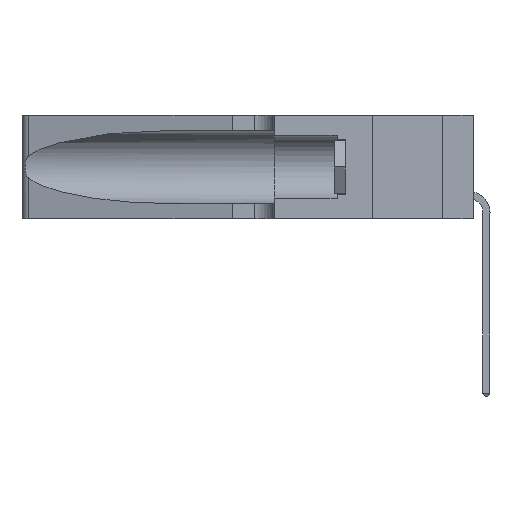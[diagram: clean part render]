
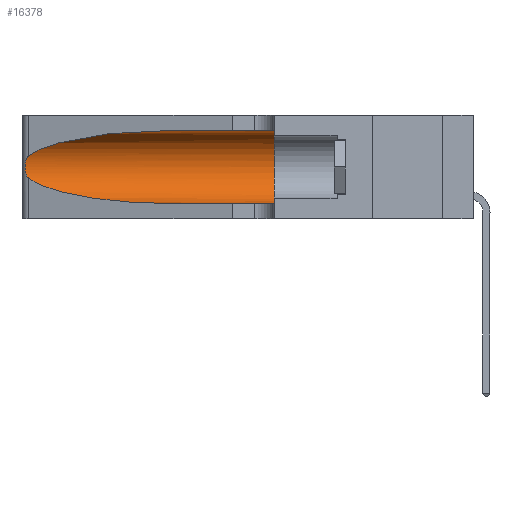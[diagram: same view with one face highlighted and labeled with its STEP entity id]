
A CAD part, left-side view. The second image highlights one B-rep face of the part: STEP entity #16378.
In plain terms, the highlighted cylindrical face has radius 3.308 mm (diameter 6.617 mm), a partial arc.
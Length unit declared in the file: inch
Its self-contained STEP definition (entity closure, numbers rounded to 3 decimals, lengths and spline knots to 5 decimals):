
#260 = DIRECTION ( 'NONE',  ( 0., -1., 0. ) ) ;
#763 = DIRECTION ( 'NONE',  ( 0., 0., 1. ) ) ;
#783 = VERTEX_POINT ( 'NONE', #12147 ) ;
#1425 = CARTESIAN_POINT ( 'NONE',  ( 0.26017, 1.23833, 0.17102 ) ) ;
#1487 = CARTESIAN_POINT ( 'NONE',  ( 0.25555, 1.22993, 0.14849 ) ) ;
#1512 = CARTESIAN_POINT ( 'NONE',  ( 0.1305, 0.72297, 0.05475 ) ) ;
#1548 = ORIENTED_EDGE ( 'NONE', *, *, #3485, .F. ) ;
#1830 = CYLINDRICAL_SURFACE ( 'NONE', #9171, 0.13025 ) ;
#1852 = EDGE_LOOP ( 'NONE', ( #7564, #5669, #13302, #5099, #1548, #5430 ) ) ;
#3246 = FACE_OUTER_BOUND ( 'NONE', #1852, .T. ) ;
#3485 = EDGE_CURVE ( 'NONE', #12063, #783, #11233, .T. ) ;
#3610 =( BOUNDED_CURVE ( )  B_SPLINE_CURVE ( 3, ( #13215, #16388, #7350, #4417 ),
 .UNSPECIFIED., .F., .F. ) 
 B_SPLINE_CURVE_WITH_KNOTS ( ( 4, 4 ),
 ( 3.44316, 4.71239 ),
 .UNSPECIFIED. ) 
 CURVE ( )  GEOMETRIC_REPRESENTATION_ITEM ( )  RATIONAL_B_SPLINE_CURVE ( ( 1., 0.87, 0.87, 1. ) ) 
 REPRESENTATION_ITEM ( '' )  );
#3836 = EDGE_CURVE ( 'NONE', #3926, #12817, #3610, .T. ) ;
#3926 = VERTEX_POINT ( 'NONE', #4865 ) ;
#4351 = CARTESIAN_POINT ( 'NONE',  ( 0.25639, 1.23184, 0.21858 ) ) ;
#4417 = CARTESIAN_POINT ( 'NONE',  ( 0.1305, 0.72297, 0.05475 ) ) ;
#4551 = CARTESIAN_POINT ( 'NONE',  ( 0.25639, 1.23186, 0.15144 ) ) ;
#4694 = CARTESIAN_POINT ( 'NONE',  ( 0.26018, 1.23835, 0.19895 ) ) ;
#4865 = CARTESIAN_POINT ( 'NONE',  ( 0.25487, 1.22718, 0.14631 ) ) ;
#5020 = VECTOR ( 'NONE', #10055, 39.37008 ) ;
#5025 = EDGE_CURVE ( 'NONE', #5330, #3926, #11076, .T. ) ;
#5099 = ORIENTED_EDGE ( 'NONE', *, *, #7749, .T. ) ;
#5251 = CARTESIAN_POINT ( 'NONE',  ( 0.1305, 1.61858, 0.185 ) ) ;
#5330 = VERTEX_POINT ( 'NONE', #8304 ) ;
#5430 = ORIENTED_EDGE ( 'NONE', *, *, #12642, .F. ) ;
#5526 = CARTESIAN_POINT ( 'NONE',  ( 0.25487, 1.22718, 0.22369 ) ) ;
#5669 = ORIENTED_EDGE ( 'NONE', *, *, #5025, .T. ) ;
#5854 = CARTESIAN_POINT ( 'NONE',  ( 0.1305, 0.72297, 0.31525 ) ) ;
#5874 = CARTESIAN_POINT ( 'NONE',  ( 0.25487, 1.22718, 0.22369 ) ) ;
#7301 = CARTESIAN_POINT ( 'NONE',  ( 0.1305, 1.61858, 0.31525 ) ) ;
#7350 = CARTESIAN_POINT ( 'NONE',  ( 0.18966, 0.96281, 0.05475 ) ) ;
#7564 = ORIENTED_EDGE ( 'NONE', *, *, #12321, .T. ) ;
#7680 = VERTEX_POINT ( 'NONE', #5854 ) ;
#7749 = EDGE_CURVE ( 'NONE', #12817, #783, #16651, .T. ) ;
#8163 = VECTOR ( 'NONE', #260, 39.37008 ) ;
#8172 = DIRECTION ( 'NONE',  ( 0., -1., 0. ) ) ;
#8304 = CARTESIAN_POINT ( 'NONE',  ( 0.25487, 1.22718, 0.22369 ) ) ;
#8635 = CARTESIAN_POINT ( 'NONE',  ( 0.25555, 1.22994, 0.2215 ) ) ;
#8955 = LINE ( 'NONE', #7301, #5020 ) ;
#9171 = AXIS2_PLACEMENT_3D ( 'NONE', #5251, #8172, #15389 ) ;
#9289 = CARTESIAN_POINT ( 'NONE',  ( 0.1305, 0.35, 0.31525 ) ) ;
#10055 = DIRECTION ( 'NONE',  ( 0., -1., 0. ) ) ;
#10503 =( BOUNDED_CURVE ( )  B_SPLINE_CURVE ( 3, ( #14374, #18672, #11238, #5526 ),
 .UNSPECIFIED., .F., .F. ) 
 B_SPLINE_CURVE_WITH_KNOTS ( ( 4, 4 ),
 ( 1.5708, 2.84003 ),
 .UNSPECIFIED. ) 
 CURVE ( )  GEOMETRIC_REPRESENTATION_ITEM ( )  RATIONAL_B_SPLINE_CURVE ( ( 1., 0.87, 0.87, 1. ) ) 
 REPRESENTATION_ITEM ( '' )  );
#10557 = CARTESIAN_POINT ( 'NONE',  ( 0.25856, 1.23593, 0.16098 ) ) ;
#11076 = B_SPLINE_CURVE_WITH_KNOTS ( 'NONE', 3,
 ( #5874, #8635, #4351, #15939, #11824, #4694, #14904, #14839, #1425, #10557, #11892, #4551, #1487, #17775 ),
 .UNSPECIFIED., .F., .F.,
 ( 4, 2, 2, 2, 2, 2, 4 ),
 ( 0., 0.00027, 0.00053, 0.00107, 0.0016, 0.00187, 0.00214 ),
 .UNSPECIFIED. ) ;
#11233 = CIRCLE ( 'NONE', #16118, 0.13025 ) ;
#11238 = CARTESIAN_POINT ( 'NONE',  ( 0.2373, 1.15595, 0.28018 ) ) ;
#11381 = CARTESIAN_POINT ( 'NONE',  ( 0.1305, 0.35, 0.185 ) ) ;
#11824 = CARTESIAN_POINT ( 'NONE',  ( 0.25854, 1.2359, 0.20912 ) ) ;
#11892 = CARTESIAN_POINT ( 'NONE',  ( 0.25789, 1.23486, 0.15765 ) ) ;
#12063 = VERTEX_POINT ( 'NONE', #9289 ) ;
#12147 = CARTESIAN_POINT ( 'NONE',  ( 0.1305, 0.35, 0.05475 ) ) ;
#12321 = EDGE_CURVE ( 'NONE', #7680, #5330, #10503, .T. ) ;
#12642 = EDGE_CURVE ( 'NONE', #7680, #12063, #8955, .T. ) ;
#12817 = VERTEX_POINT ( 'NONE', #1512 ) ;
#13215 = CARTESIAN_POINT ( 'NONE',  ( 0.25487, 1.22718, 0.14631 ) ) ;
#13302 = ORIENTED_EDGE ( 'NONE', *, *, #3836, .T. ) ;
#13591 = CARTESIAN_POINT ( 'NONE',  ( 0.1305, 1.61858, 0.05475 ) ) ;
#14374 = CARTESIAN_POINT ( 'NONE',  ( 0.1305, 0.72297, 0.31525 ) ) ;
#14839 = CARTESIAN_POINT ( 'NONE',  ( 0.26075, 1.23896, 0.178 ) ) ;
#14904 = CARTESIAN_POINT ( 'NONE',  ( 0.26075, 1.23896, 0.19203 ) ) ;
#15389 = DIRECTION ( 'NONE',  ( 0., 0., -1. ) ) ;
#15939 = CARTESIAN_POINT ( 'NONE',  ( 0.25787, 1.23484, 0.2124 ) ) ;
#16118 = AXIS2_PLACEMENT_3D ( 'NONE', #11381, #18676, #763 ) ;
#16378 = ADVANCED_FACE ( 'NONE', ( #3246 ), #1830, .F. ) ;
#16388 = CARTESIAN_POINT ( 'NONE',  ( 0.2373, 1.15595, 0.08982 ) ) ;
#16651 = LINE ( 'NONE', #13591, #8163 ) ;
#17775 = CARTESIAN_POINT ( 'NONE',  ( 0.25487, 1.22718, 0.14631 ) ) ;
#18672 = CARTESIAN_POINT ( 'NONE',  ( 0.18966, 0.96281, 0.31525 ) ) ;
#18676 = DIRECTION ( 'NONE',  ( 0., 1., 0. ) ) ;
